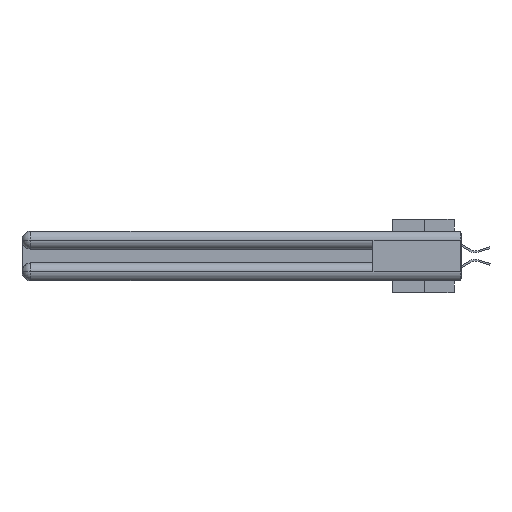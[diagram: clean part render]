
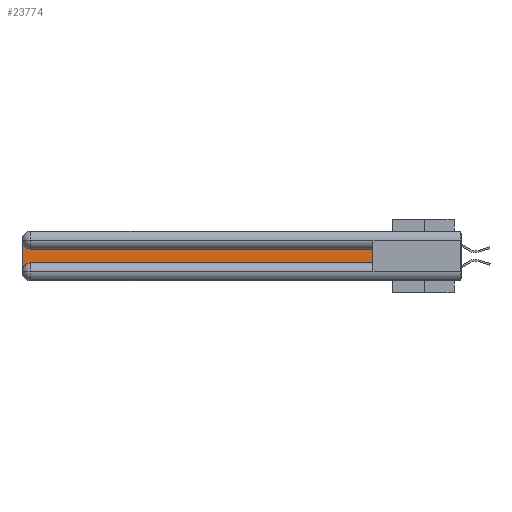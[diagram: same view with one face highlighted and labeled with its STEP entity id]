
A CAD part, left-side view. The second image highlights one B-rep face of the part: STEP entity #23774.
In plain terms, the highlighted planar face has unit normal (-1, 0, 0).
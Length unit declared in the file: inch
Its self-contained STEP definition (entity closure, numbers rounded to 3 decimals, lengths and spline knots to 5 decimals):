
#513 = VERTEX_POINT ( 'NONE', #26027 ) ;
#636 = ORIENTED_EDGE ( 'NONE', *, *, #7382, .T. ) ;
#1042 = DIRECTION ( 'NONE',  ( 0., 1., 0. ) ) ;
#2145 = EDGE_CURVE ( 'NONE', #15000, #4893, #12725, .T. ) ;
#2524 = CIRCLE ( 'NONE', #18773, 0.06 ) ;
#3018 = CARTESIAN_POINT ( 'NONE',  ( 0.075, 3., -0.1225 ) ) ;
#3024 = DIRECTION ( 'NONE',  ( 1., 0., 0. ) ) ;
#3574 = CARTESIAN_POINT ( 'NONE',  ( 0.075, 0.6, -0.1225 ) ) ;
#4893 = VERTEX_POINT ( 'NONE', #21076 ) ;
#4912 = CARTESIAN_POINT ( 'NONE',  ( 0.075, 0.6, -0.2175 ) ) ;
#5136 = VERTEX_POINT ( 'NONE', #15327 ) ;
#6456 = EDGE_LOOP ( 'NONE', ( #19023, #21322, #27433, #31533, #16888, #636 ) ) ;
#7382 = EDGE_CURVE ( 'NONE', #4893, #21737, #12290, .T. ) ;
#7500 = CARTESIAN_POINT ( 'NONE',  ( 0.075, 3., -0.2175 ) ) ;
#7863 = AXIS2_PLACEMENT_3D ( 'NONE', #22863, #3024, #10428 ) ;
#8109 = PLANE ( 'NONE',  #24584 ) ;
#8400 = CARTESIAN_POINT ( 'NONE',  ( 0.075, 2.94, -0.0625 ) ) ;
#9681 = DIRECTION ( 'NONE',  ( 0., 0., 1. ) ) ;
#10274 = CARTESIAN_POINT ( 'NONE',  ( 0.075, 0.6, -0.2175 ) ) ;
#10428 = DIRECTION ( 'NONE',  ( 0., 0., -1. ) ) ;
#10605 = DIRECTION ( 'NONE',  ( 0., -1., 0. ) ) ;
#11079 = EDGE_CURVE ( 'NONE', #21737, #5136, #16304, .T. ) ;
#11918 = VECTOR ( 'NONE', #10605, 39.37008 ) ;
#12260 = DIRECTION ( 'NONE',  ( 0., 0., -1. ) ) ;
#12290 = LINE ( 'NONE', #4912, #12811 ) ;
#12724 = EDGE_CURVE ( 'NONE', #5136, #17578, #2524, .T. ) ;
#12725 = LINE ( 'NONE', #10274, #11918 ) ;
#12811 = VECTOR ( 'NONE', #9681, 39.37008 ) ;
#15000 = VERTEX_POINT ( 'NONE', #16347 ) ;
#15327 = CARTESIAN_POINT ( 'NONE',  ( 0.075, 2.94, -0.1225 ) ) ;
#15697 = CIRCLE ( 'NONE', #7863, 0.06 ) ;
#16304 = LINE ( 'NONE', #23513, #30291 ) ;
#16347 = CARTESIAN_POINT ( 'NONE',  ( 0.075, 2.94, -0.2175 ) ) ;
#16888 = ORIENTED_EDGE ( 'NONE', *, *, #2145, .T. ) ;
#17453 = DIRECTION ( 'NONE',  ( 1., 0., 0. ) ) ;
#17547 = EDGE_CURVE ( 'NONE', #17578, #513, #29350, .T. ) ;
#17578 = VERTEX_POINT ( 'NONE', #27014 ) ;
#18705 = DIRECTION ( 'NONE',  ( 1., 0., 0. ) ) ;
#18773 = AXIS2_PLACEMENT_3D ( 'NONE', #8400, #18705, #26256 ) ;
#19023 = ORIENTED_EDGE ( 'NONE', *, *, #11079, .T. ) ;
#21076 = CARTESIAN_POINT ( 'NONE',  ( 0.075, 0.6, -0.2175 ) ) ;
#21322 = ORIENTED_EDGE ( 'NONE', *, *, #12724, .T. ) ;
#21737 = VERTEX_POINT ( 'NONE', #3574 ) ;
#22863 = CARTESIAN_POINT ( 'NONE',  ( 0.075, 2.94, -0.2775 ) ) ;
#23513 = CARTESIAN_POINT ( 'NONE',  ( 0.075, 0.6, -0.1225 ) ) ;
#23774 = ADVANCED_FACE ( 'NONE', ( #28123 ), #8109, .F. ) ;
#24584 = AXIS2_PLACEMENT_3D ( 'NONE', #3018, #17453, #27632 ) ;
#26027 = CARTESIAN_POINT ( 'NONE',  ( 0.075, 3., -0.2775 ) ) ;
#26256 = DIRECTION ( 'NONE',  ( 0., 0., -1. ) ) ;
#27014 = CARTESIAN_POINT ( 'NONE',  ( 0.075, 3., -0.0625 ) ) ;
#27433 = ORIENTED_EDGE ( 'NONE', *, *, #17547, .T. ) ;
#27495 = VECTOR ( 'NONE', #12260, 39.37008 ) ;
#27632 = DIRECTION ( 'NONE',  ( 0., 0., -1. ) ) ;
#28123 = FACE_OUTER_BOUND ( 'NONE', #6456, .T. ) ;
#29350 = LINE ( 'NONE', #7500, #27495 ) ;
#30291 = VECTOR ( 'NONE', #1042, 39.37008 ) ;
#31533 = ORIENTED_EDGE ( 'NONE', *, *, #31611, .T. ) ;
#31611 = EDGE_CURVE ( 'NONE', #513, #15000, #15697, .T. ) ;
